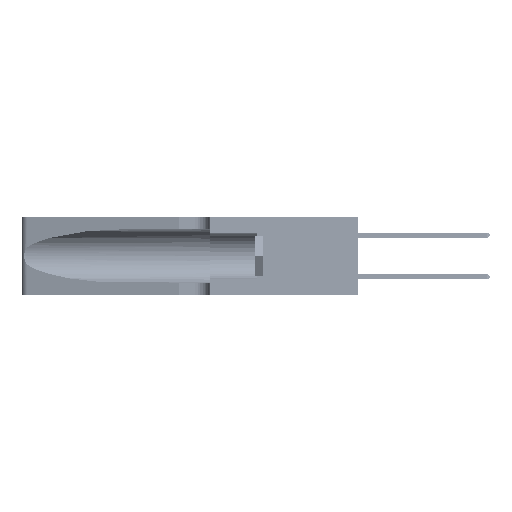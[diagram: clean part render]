
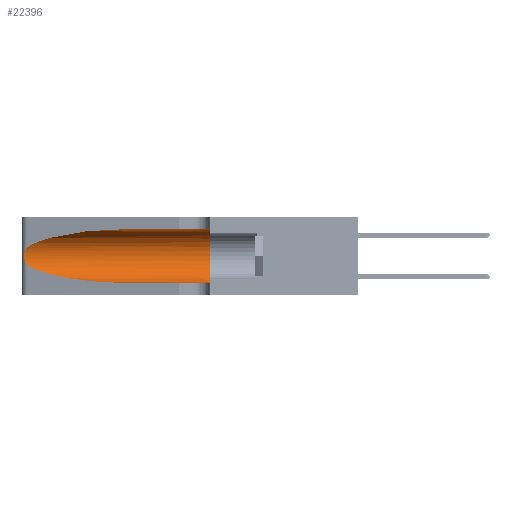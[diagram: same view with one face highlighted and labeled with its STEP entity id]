
A CAD part, left-side view. The second image highlights one B-rep face of the part: STEP entity #22396.
In plain terms, the highlighted cylindrical face has radius 3.308 mm (diameter 6.617 mm), a partial arc.
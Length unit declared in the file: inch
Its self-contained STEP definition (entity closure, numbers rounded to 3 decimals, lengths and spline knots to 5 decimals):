
#133 = CARTESIAN_POINT ( 'NONE',  ( 0.1305, 0.72297, 0.05475 ) ) ;
#677 = DIRECTION ( 'NONE',  ( 0., 0., -1. ) ) ;
#844 = EDGE_CURVE ( 'NONE', #49220, #26613, #21869, .T. ) ;
#3191 = CARTESIAN_POINT ( 'NONE',  ( 0.25639, 1.23184, 0.21858 ) ) ;
#3605 = ORIENTED_EDGE ( 'NONE', *, *, #844, .T. ) ;
#5253 = VERTEX_POINT ( 'NONE', #48807 ) ;
#5493 =( BOUNDED_CURVE ( )  B_SPLINE_CURVE ( 3, ( #17271, #50871, #25782, #133 ),
 .UNSPECIFIED., .F., .F. ) 
 B_SPLINE_CURVE_WITH_KNOTS ( ( 4, 4 ),
 ( 3.44316, 4.71239 ),
 .UNSPECIFIED. ) 
 CURVE ( )  GEOMETRIC_REPRESENTATION_ITEM ( )  RATIONAL_B_SPLINE_CURVE ( ( 1., 0.87, 0.87, 1. ) ) 
 REPRESENTATION_ITEM ( '' )  );
#7573 = CARTESIAN_POINT ( 'NONE',  ( 0.25854, 1.2359, 0.20912 ) ) ;
#7866 = DIRECTION ( 'NONE',  ( 0., 1., 0. ) ) ;
#8335 = ORIENTED_EDGE ( 'NONE', *, *, #46781, .T. ) ;
#8522 = CARTESIAN_POINT ( 'NONE',  ( 0.2373, 1.15595, 0.28018 ) ) ;
#9284 = CARTESIAN_POINT ( 'NONE',  ( 0.1305, 1.61858, 0.31525 ) ) ;
#9635 = LINE ( 'NONE', #9284, #43840 ) ;
#10525 = VECTOR ( 'NONE', #30359, 39.37008 ) ;
#11794 = EDGE_CURVE ( 'NONE', #5253, #13069, #19594, .T. ) ;
#11861 = CARTESIAN_POINT ( 'NONE',  ( 0.26075, 1.23896, 0.19203 ) ) ;
#12436 = VERTEX_POINT ( 'NONE', #25017 ) ;
#13069 = VERTEX_POINT ( 'NONE', #24955 ) ;
#13556 = DIRECTION ( 'NONE',  ( 0., -1., 0. ) ) ;
#13725 = CYLINDRICAL_SURFACE ( 'NONE', #20170, 0.13025 ) ;
#16171 = CARTESIAN_POINT ( 'NONE',  ( 0.26017, 1.23833, 0.17102 ) ) ;
#16504 = CARTESIAN_POINT ( 'NONE',  ( 0.1305, 0.35, 0.31525 ) ) ;
#17271 = CARTESIAN_POINT ( 'NONE',  ( 0.25487, 1.22718, 0.14631 ) ) ;
#19594 = B_SPLINE_CURVE_WITH_KNOTS ( 'NONE', 3,
 ( #24528, #28752, #3191, #32964, #7573, #37194, #11861, #41423, #16171, #45609, #20460, #49810, #24708, #53988 ),
 .UNSPECIFIED., .F., .F.,
 ( 4, 2, 2, 2, 2, 2, 4 ),
 ( 0., 0.00027, 0.00053, 0.00107, 0.0016, 0.00187, 0.00214 ),
 .UNSPECIFIED. ) ;
#20170 = AXIS2_PLACEMENT_3D ( 'NONE', #26306, #43013, #677 ) ;
#20330 = VERTEX_POINT ( 'NONE', #16504 ) ;
#20460 = CARTESIAN_POINT ( 'NONE',  ( 0.25789, 1.23486, 0.15765 ) ) ;
#21869 = LINE ( 'NONE', #42861, #10525 ) ;
#22396 = ADVANCED_FACE ( 'NONE', ( #26367 ), #13725, .F. ) ;
#23290 = CIRCLE ( 'NONE', #49186, 0.13025 ) ;
#24528 = CARTESIAN_POINT ( 'NONE',  ( 0.25487, 1.22718, 0.22369 ) ) ;
#24708 = CARTESIAN_POINT ( 'NONE',  ( 0.25555, 1.22993, 0.14849 ) ) ;
#24955 = CARTESIAN_POINT ( 'NONE',  ( 0.25487, 1.22718, 0.14631 ) ) ;
#25004 = ORIENTED_EDGE ( 'NONE', *, *, #42729, .T. ) ;
#25017 = CARTESIAN_POINT ( 'NONE',  ( 0.1305, 0.72297, 0.31525 ) ) ;
#25465 = CARTESIAN_POINT ( 'NONE',  ( 0.18966, 0.96281, 0.31525 ) ) ;
#25782 = CARTESIAN_POINT ( 'NONE',  ( 0.18966, 0.96281, 0.05475 ) ) ;
#26306 = CARTESIAN_POINT ( 'NONE',  ( 0.1305, 1.61858, 0.185 ) ) ;
#26367 = FACE_OUTER_BOUND ( 'NONE', #46292, .T. ) ;
#26613 = VERTEX_POINT ( 'NONE', #49583 ) ;
#28752 = CARTESIAN_POINT ( 'NONE',  ( 0.25555, 1.22994, 0.2215 ) ) ;
#30270 = ORIENTED_EDGE ( 'NONE', *, *, #47611, .F. ) ;
#30359 = DIRECTION ( 'NONE',  ( 0., -1., 0. ) ) ;
#32964 = CARTESIAN_POINT ( 'NONE',  ( 0.25787, 1.23484, 0.2124 ) ) ;
#33271 = CARTESIAN_POINT ( 'NONE',  ( 0.1305, 0.35, 0.185 ) ) ;
#36878 = ORIENTED_EDGE ( 'NONE', *, *, #51555, .F. ) ;
#37194 = CARTESIAN_POINT ( 'NONE',  ( 0.26018, 1.23835, 0.19895 ) ) ;
#37500 = DIRECTION ( 'NONE',  ( 0., 0., 1. ) ) ;
#38159 = CARTESIAN_POINT ( 'NONE',  ( 0.25487, 1.22718, 0.22369 ) ) ;
#39575 = CARTESIAN_POINT ( 'NONE',  ( 0.1305, 0.72297, 0.05475 ) ) ;
#40843 =( BOUNDED_CURVE ( )  B_SPLINE_CURVE ( 3, ( #54754, #25465, #8522, #38159 ),
 .UNSPECIFIED., .F., .T. ) 
 B_SPLINE_CURVE_WITH_KNOTS ( ( 4, 4 ),
 ( 1.5708, 2.84003 ),
 .UNSPECIFIED. ) 
 CURVE ( )  GEOMETRIC_REPRESENTATION_ITEM ( )  RATIONAL_B_SPLINE_CURVE ( ( 1., 0.87, 0.87, 1. ) ) 
 REPRESENTATION_ITEM ( '' )  );
#41423 = CARTESIAN_POINT ( 'NONE',  ( 0.26075, 1.23896, 0.178 ) ) ;
#42729 = EDGE_CURVE ( 'NONE', #13069, #49220, #5493, .T. ) ;
#42861 = CARTESIAN_POINT ( 'NONE',  ( 0.1305, 1.61858, 0.05475 ) ) ;
#43013 = DIRECTION ( 'NONE',  ( 0., -1., 0. ) ) ;
#43840 = VECTOR ( 'NONE', #13556, 39.37008 ) ;
#45609 = CARTESIAN_POINT ( 'NONE',  ( 0.25856, 1.23593, 0.16098 ) ) ;
#46292 = EDGE_LOOP ( 'NONE', ( #8335, #53174, #25004, #3605, #30270, #36878 ) ) ;
#46781 = EDGE_CURVE ( 'NONE', #12436, #5253, #40843, .T. ) ;
#47611 = EDGE_CURVE ( 'NONE', #20330, #26613, #23290, .T. ) ;
#48807 = CARTESIAN_POINT ( 'NONE',  ( 0.25487, 1.22718, 0.22369 ) ) ;
#49186 = AXIS2_PLACEMENT_3D ( 'NONE', #33271, #7866, #37500 ) ;
#49220 = VERTEX_POINT ( 'NONE', #39575 ) ;
#49583 = CARTESIAN_POINT ( 'NONE',  ( 0.1305, 0.35, 0.05475 ) ) ;
#49810 = CARTESIAN_POINT ( 'NONE',  ( 0.25639, 1.23186, 0.15144 ) ) ;
#50871 = CARTESIAN_POINT ( 'NONE',  ( 0.2373, 1.15595, 0.08982 ) ) ;
#51555 = EDGE_CURVE ( 'NONE', #12436, #20330, #9635, .T. ) ;
#53174 = ORIENTED_EDGE ( 'NONE', *, *, #11794, .T. ) ;
#53988 = CARTESIAN_POINT ( 'NONE',  ( 0.25487, 1.22718, 0.14631 ) ) ;
#54754 = CARTESIAN_POINT ( 'NONE',  ( 0.1305, 0.72297, 0.31525 ) ) ;
